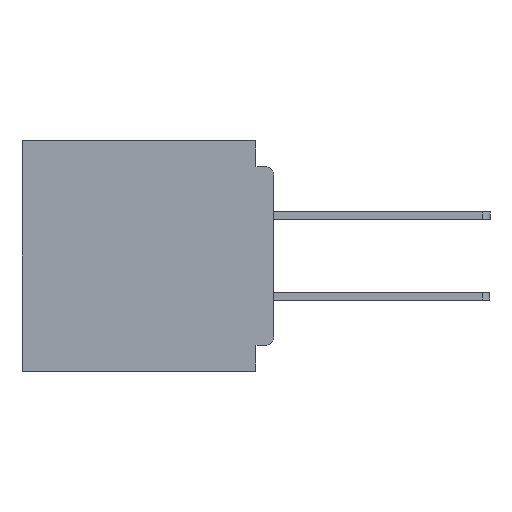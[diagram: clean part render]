
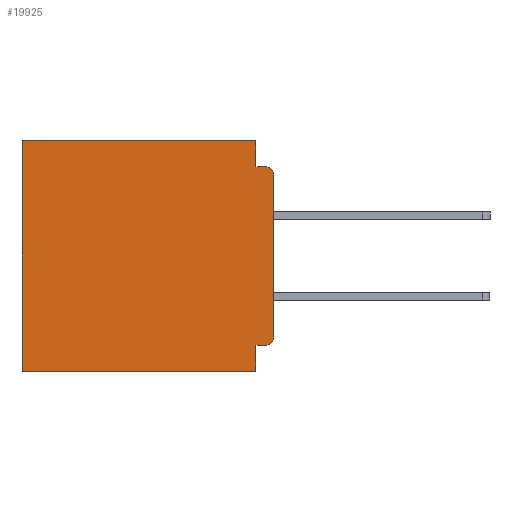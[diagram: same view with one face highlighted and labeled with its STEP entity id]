
A CAD part, left-side view. The second image highlights one B-rep face of the part: STEP entity #19925.
In plain terms, the highlighted planar face has unit normal (-1, 0, 0).
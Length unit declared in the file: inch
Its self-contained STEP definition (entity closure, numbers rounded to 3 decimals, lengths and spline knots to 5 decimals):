
#1020 = EDGE_CURVE ( 'NONE', #16085, #18445, #9938, .T. ) ;
#1079 = EDGE_CURVE ( 'NONE', #18680, #21116, #31837, .T. ) ;
#1317 = LINE ( 'NONE', #17190, #24357 ) ;
#2346 = DIRECTION ( 'NONE',  ( 0., 0., -1. ) ) ;
#2512 = VECTOR ( 'NONE', #15008, 39.37008 ) ;
#2515 = LINE ( 'NONE', #17321, #24565 ) ;
#2581 = EDGE_CURVE ( 'NONE', #19412, #18445, #34047, .T. ) ;
#5222 = CARTESIAN_POINT ( 'NONE',  ( 0.3, 0., -0.045 ) ) ;
#5561 = EDGE_CURVE ( 'NONE', #20844, #15292, #10536, .T. ) ;
#5708 = CARTESIAN_POINT ( 'NONE',  ( 0.3, 0., -0.4 ) ) ;
#5847 = EDGE_CURVE ( 'NONE', #28569, #24035, #31935, .T. ) ;
#5933 = CARTESIAN_POINT ( 'NONE',  ( 0.3, 0.437, 0. ) ) ;
#6097 = DIRECTION ( 'NONE',  ( 0., -1., 0. ) ) ;
#6277 = ORIENTED_EDGE ( 'NONE', *, *, #21735, .F. ) ;
#7322 = CARTESIAN_POINT ( 'NONE',  ( 0.3, 0.031, 0. ) ) ;
#8598 = DIRECTION ( 'NONE',  ( 0., 0., -1. ) ) ;
#8641 = ORIENTED_EDGE ( 'NONE', *, *, #1020, .F. ) ;
#9319 = LINE ( 'NONE', #38193, #32181 ) ;
#9938 = LINE ( 'NONE', #13589, #24894 ) ;
#10536 = LINE ( 'NONE', #16431, #2512 ) ;
#10920 = EDGE_LOOP ( 'NONE', ( #8641, #11497, #16145, #6277, #22715, #21304, #31533, #37067, #16182, #24598 ) ) ;
#11497 = ORIENTED_EDGE ( 'NONE', *, *, #12680, .T. ) ;
#12043 = CARTESIAN_POINT ( 'NONE',  ( 0.3, 0., -0.4 ) ) ;
#12680 = EDGE_CURVE ( 'NONE', #16085, #24035, #34050, .T. ) ;
#13339 = CARTESIAN_POINT ( 'NONE',  ( 0.3, 0.015, -0.06 ) ) ;
#13589 = CARTESIAN_POINT ( 'NONE',  ( 0.3, 0., -0.4 ) ) ;
#13653 = CARTESIAN_POINT ( 'NONE',  ( 0.3, 0.437, -0.4 ) ) ;
#13918 = VECTOR ( 'NONE', #29637, 39.37008 ) ;
#14697 = CARTESIAN_POINT ( 'NONE',  ( 0.3, 0.031, -0.4 ) ) ;
#14954 = CARTESIAN_POINT ( 'NONE',  ( 0.3, 0.015, -0.355 ) ) ;
#15008 = DIRECTION ( 'NONE',  ( 0., 1., 0. ) ) ;
#15105 = VECTOR ( 'NONE', #37337, 39.37008 ) ;
#15292 = VERTEX_POINT ( 'NONE', #5933 ) ;
#15707 = AXIS2_PLACEMENT_3D ( 'NONE', #15847, #32749, #2346 ) ;
#15775 = LINE ( 'NONE', #5708, #13918 ) ;
#15847 = CARTESIAN_POINT ( 'NONE',  ( 0.3, 0.015, -0.34 ) ) ;
#16085 = VERTEX_POINT ( 'NONE', #21721 ) ;
#16102 = VECTOR ( 'NONE', #6097, 39.37008 ) ;
#16145 = ORIENTED_EDGE ( 'NONE', *, *, #5847, .F. ) ;
#16182 = ORIENTED_EDGE ( 'NONE', *, *, #22669, .F. ) ;
#16278 = DIRECTION ( 'NONE',  ( 0., 0., -1. ) ) ;
#16431 = CARTESIAN_POINT ( 'NONE',  ( 0.3, 0., 0. ) ) ;
#16886 = FACE_OUTER_BOUND ( 'NONE', #10920, .T. ) ;
#17190 = CARTESIAN_POINT ( 'NONE',  ( 0.3, 0., -0.355 ) ) ;
#17321 = CARTESIAN_POINT ( 'NONE',  ( 0.3, 0.437, -0.4 ) ) ;
#17898 = EDGE_CURVE ( 'NONE', #15292, #32200, #2515, .T. ) ;
#17998 = DIRECTION ( 'NONE',  ( 1., 0., 0. ) ) ;
#18445 = VERTEX_POINT ( 'NONE', #19898 ) ;
#18462 = CARTESIAN_POINT ( 'NONE',  ( 0.3, 0.031, -0.045 ) ) ;
#18680 = VERTEX_POINT ( 'NONE', #29920 ) ;
#19412 = VERTEX_POINT ( 'NONE', #14954 ) ;
#19898 = CARTESIAN_POINT ( 'NONE',  ( 0.3, 0., -0.34 ) ) ;
#19925 = ADVANCED_FACE ( 'NONE', ( #16886 ), #35794, .F. ) ;
#20494 = CARTESIAN_POINT ( 'NONE',  ( 0.3, 0.015, -0.045 ) ) ;
#20844 = VERTEX_POINT ( 'NONE', #7322 ) ;
#21116 = VERTEX_POINT ( 'NONE', #14697 ) ;
#21304 = ORIENTED_EDGE ( 'NONE', *, *, #17898, .T. ) ;
#21721 = CARTESIAN_POINT ( 'NONE',  ( 0.3, 0., -0.06 ) ) ;
#21735 = EDGE_CURVE ( 'NONE', #20844, #28569, #9319, .T. ) ;
#22669 = EDGE_CURVE ( 'NONE', #19412, #18680, #1317, .T. ) ;
#22715 = ORIENTED_EDGE ( 'NONE', *, *, #5561, .T. ) ;
#22973 = AXIS2_PLACEMENT_3D ( 'NONE', #13339, #34128, #16278 ) ;
#24035 = VERTEX_POINT ( 'NONE', #20494 ) ;
#24357 = VECTOR ( 'NONE', #35000, 39.37008 ) ;
#24565 = VECTOR ( 'NONE', #26355, 39.37008 ) ;
#24598 = ORIENTED_EDGE ( 'NONE', *, *, #2581, .T. ) ;
#24894 = VECTOR ( 'NONE', #30978, 39.37008 ) ;
#26355 = DIRECTION ( 'NONE',  ( 0., 0., -1. ) ) ;
#28569 = VERTEX_POINT ( 'NONE', #18462 ) ;
#29044 = EDGE_CURVE ( 'NONE', #21116, #32200, #15775, .T. ) ;
#29637 = DIRECTION ( 'NONE',  ( 0., 1., 0. ) ) ;
#29920 = CARTESIAN_POINT ( 'NONE',  ( 0.3, 0.031, -0.355 ) ) ;
#30978 = DIRECTION ( 'NONE',  ( 0., 0., -1. ) ) ;
#31533 = ORIENTED_EDGE ( 'NONE', *, *, #29044, .F. ) ;
#31837 = LINE ( 'NONE', #36289, #15105 ) ;
#31935 = LINE ( 'NONE', #5222, #16102 ) ;
#32181 = VECTOR ( 'NONE', #8598, 39.37008 ) ;
#32200 = VERTEX_POINT ( 'NONE', #13653 ) ;
#32749 = DIRECTION ( 'NONE',  ( -1., 0., 0. ) ) ;
#33093 = AXIS2_PLACEMENT_3D ( 'NONE', #12043, #17998, #38715 ) ;
#34047 = CIRCLE ( 'NONE', #15707, 0.015 ) ;
#34050 = CIRCLE ( 'NONE', #22973, 0.015 ) ;
#34128 = DIRECTION ( 'NONE',  ( -1., 0., 0. ) ) ;
#35000 = DIRECTION ( 'NONE',  ( 0., 1., 0. ) ) ;
#35794 = PLANE ( 'NONE',  #33093 ) ;
#36289 = CARTESIAN_POINT ( 'NONE',  ( 0.3, 0.031, -0.4 ) ) ;
#37067 = ORIENTED_EDGE ( 'NONE', *, *, #1079, .F. ) ;
#37337 = DIRECTION ( 'NONE',  ( 0., 0., -1. ) ) ;
#38193 = CARTESIAN_POINT ( 'NONE',  ( 0.3, 0.031, 0. ) ) ;
#38715 = DIRECTION ( 'NONE',  ( 0., 0., -1. ) ) ;
